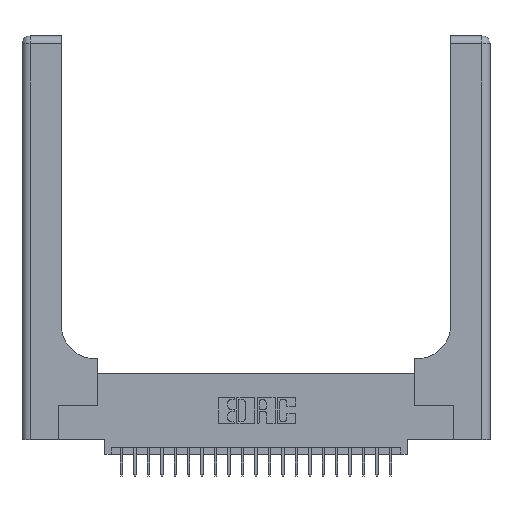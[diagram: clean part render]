
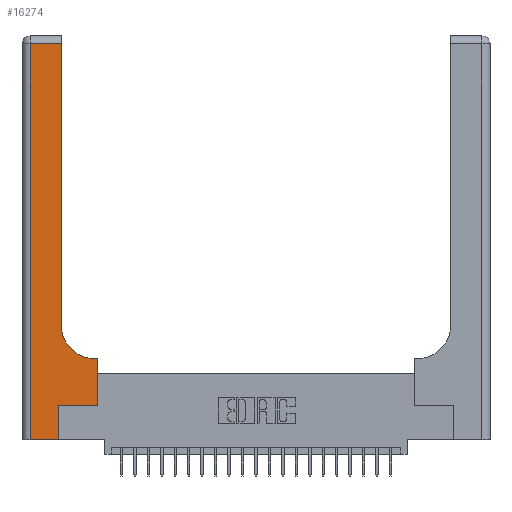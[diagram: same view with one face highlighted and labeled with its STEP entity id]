
A CAD part, top view. The second image highlights one B-rep face of the part: STEP entity #16274.
In plain terms, the highlighted planar face has unit normal (0, 0, 1).
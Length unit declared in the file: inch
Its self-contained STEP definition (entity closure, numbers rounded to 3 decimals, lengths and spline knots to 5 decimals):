
#888 = VERTEX_POINT ( 'NONE', #21988 ) ;
#1261 = VERTEX_POINT ( 'NONE', #2421 ) ;
#1619 = ORIENTED_EDGE ( 'NONE', *, *, #13342, .T. ) ;
#1737 = PLANE ( 'NONE',  #21471 ) ;
#1777 = ORIENTED_EDGE ( 'NONE', *, *, #7216, .T. ) ;
#1862 = VECTOR ( 'NONE', #7499, 39.37008 ) ;
#1919 = DIRECTION ( 'NONE',  ( 1., 0., 0. ) ) ;
#2384 = CARTESIAN_POINT ( 'NONE',  ( 0.5415, 0.85, 0.37 ) ) ;
#2421 = CARTESIAN_POINT ( 'NONE',  ( 0.2915, 0.85, 0.37 ) ) ;
#2678 = LINE ( 'NONE', #13733, #18095 ) ;
#3029 = DIRECTION ( 'NONE',  ( -1., 0., 0. ) ) ;
#3164 = DIRECTION ( 'NONE',  ( -1., 0., 0. ) ) ;
#3308 = DIRECTION ( 'NONE',  ( 1., 0., 0. ) ) ;
#3447 = EDGE_CURVE ( 'NONE', #16930, #23246, #9148, .T. ) ;
#3741 = LINE ( 'NONE', #9834, #22646 ) ;
#3950 = LINE ( 'NONE', #16737, #19202 ) ;
#4475 = DIRECTION ( 'NONE',  ( 1., 0., 0. ) ) ;
#4646 = EDGE_CURVE ( 'NONE', #7047, #4880, #20685, .T. ) ;
#4851 = ORIENTED_EDGE ( 'NONE', *, *, #3447, .T. ) ;
#4880 = VERTEX_POINT ( 'NONE', #11845 ) ;
#5863 = CARTESIAN_POINT ( 'NONE',  ( 0., 3., 0.37 ) ) ;
#6146 = AXIS2_PLACEMENT_3D ( 'NONE', #2384, #16051, #4475 ) ;
#7047 = VERTEX_POINT ( 'NONE', #7310 ) ;
#7190 = CARTESIAN_POINT ( 'NONE',  ( 0.269, 0.25, 0.37 ) ) ;
#7216 = EDGE_CURVE ( 'NONE', #1261, #16674, #3741, .T. ) ;
#7310 = CARTESIAN_POINT ( 'NONE',  ( 0.06, 2.94, 0.37 ) ) ;
#7315 = ORIENTED_EDGE ( 'NONE', *, *, #13772, .T. ) ;
#7499 = DIRECTION ( 'NONE',  ( 0., 1., 0. ) ) ;
#7893 = EDGE_LOOP ( 'NONE', ( #1777, #7315, #17401, #1619, #4851, #12731, #19799, #12259, #16457 ) ) ;
#7895 = DIRECTION ( 'NONE',  ( -1., 0., 0. ) ) ;
#8299 = LINE ( 'NONE', #9039, #12201 ) ;
#8674 = EDGE_CURVE ( 'NONE', #11472, #1261, #23148, .T. ) ;
#9024 = VERTEX_POINT ( 'NONE', #18934 ) ;
#9039 = CARTESIAN_POINT ( 'NONE',  ( 0.2915, 0.6, 0.37 ) ) ;
#9148 = LINE ( 'NONE', #15069, #1862 ) ;
#9645 = VECTOR ( 'NONE', #3308, 39.37008 ) ;
#9834 = CARTESIAN_POINT ( 'NONE',  ( 0.2915, 3., 0.37 ) ) ;
#9995 = LINE ( 'NONE', #12053, #19298 ) ;
#10301 = VECTOR ( 'NONE', #22146, 39.37008 ) ;
#11472 = VERTEX_POINT ( 'NONE', #13287 ) ;
#11845 = CARTESIAN_POINT ( 'NONE',  ( 0.06, 0., 0.37 ) ) ;
#12053 = CARTESIAN_POINT ( 'NONE',  ( 0.5585, 0.25, 0.37 ) ) ;
#12201 = VECTOR ( 'NONE', #3029, 39.37008 ) ;
#12259 = ORIENTED_EDGE ( 'NONE', *, *, #15510, .T. ) ;
#12604 = EDGE_CURVE ( 'NONE', #23246, #888, #23721, .T. ) ;
#12731 = ORIENTED_EDGE ( 'NONE', *, *, #12604, .T. ) ;
#13080 = CARTESIAN_POINT ( 'NONE',  ( 0.06, 3., 0.37 ) ) ;
#13287 = CARTESIAN_POINT ( 'NONE',  ( 0.5415, 0.6, 0.37 ) ) ;
#13342 = EDGE_CURVE ( 'NONE', #4880, #16930, #2678, .T. ) ;
#13733 = CARTESIAN_POINT ( 'NONE',  ( 0., 0., 0.37 ) ) ;
#13772 = EDGE_CURVE ( 'NONE', #16674, #7047, #3950, .T. ) ;
#14990 = CARTESIAN_POINT ( 'NONE',  ( 0.269, 0.25, 0.37 ) ) ;
#15069 = CARTESIAN_POINT ( 'NONE',  ( 0.269, 0., 0.37 ) ) ;
#15510 = EDGE_CURVE ( 'NONE', #9024, #11472, #8299, .T. ) ;
#15794 = DIRECTION ( 'NONE',  ( 0., 1., 0. ) ) ;
#16051 = DIRECTION ( 'NONE',  ( 0., 0., -1. ) ) ;
#16274 = ADVANCED_FACE ( 'NONE', ( #24668 ), #1737, .F. ) ;
#16457 = ORIENTED_EDGE ( 'NONE', *, *, #8674, .T. ) ;
#16674 = VERTEX_POINT ( 'NONE', #22144 ) ;
#16737 = CARTESIAN_POINT ( 'NONE',  ( 0., 2.94, 0.37 ) ) ;
#16930 = VERTEX_POINT ( 'NONE', #17364 ) ;
#17364 = CARTESIAN_POINT ( 'NONE',  ( 0.269, 0., 0.37 ) ) ;
#17390 = DIRECTION ( 'NONE',  ( 0., 1., 0. ) ) ;
#17401 = ORIENTED_EDGE ( 'NONE', *, *, #4646, .T. ) ;
#17680 = EDGE_CURVE ( 'NONE', #888, #9024, #9995, .T. ) ;
#18095 = VECTOR ( 'NONE', #1919, 39.37008 ) ;
#18934 = CARTESIAN_POINT ( 'NONE',  ( 0.5585, 0.6, 0.37 ) ) ;
#19120 = DIRECTION ( 'NONE',  ( 0., 0., -1. ) ) ;
#19202 = VECTOR ( 'NONE', #3164, 39.37008 ) ;
#19298 = VECTOR ( 'NONE', #15794, 39.37008 ) ;
#19799 = ORIENTED_EDGE ( 'NONE', *, *, #17680, .T. ) ;
#20685 = LINE ( 'NONE', #13080, #10301 ) ;
#21471 = AXIS2_PLACEMENT_3D ( 'NONE', #5863, #19120, #7895 ) ;
#21988 = CARTESIAN_POINT ( 'NONE',  ( 0.5585, 0.25, 0.37 ) ) ;
#22144 = CARTESIAN_POINT ( 'NONE',  ( 0.2915, 2.94, 0.37 ) ) ;
#22146 = DIRECTION ( 'NONE',  ( 0., -1., 0. ) ) ;
#22646 = VECTOR ( 'NONE', #17390, 39.37008 ) ;
#23148 = CIRCLE ( 'NONE', #6146, 0.25 ) ;
#23246 = VERTEX_POINT ( 'NONE', #7190 ) ;
#23721 = LINE ( 'NONE', #14990, #9645 ) ;
#24668 = FACE_OUTER_BOUND ( 'NONE', #7893, .T. ) ;
